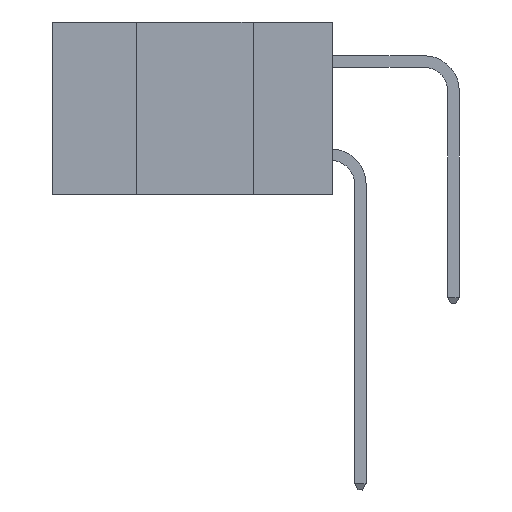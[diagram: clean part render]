
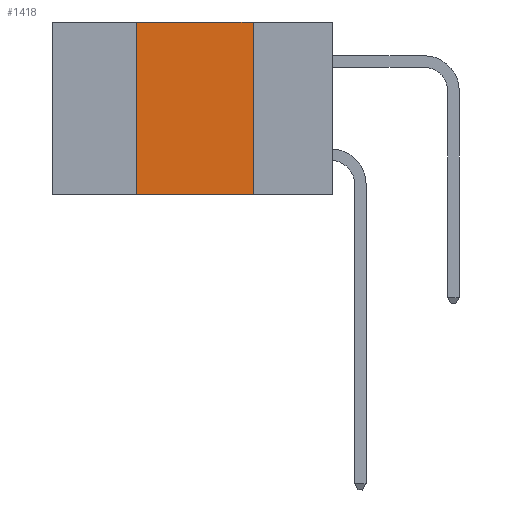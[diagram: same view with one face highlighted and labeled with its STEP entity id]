
A CAD part, left-side view. The second image highlights one B-rep face of the part: STEP entity #1418.
In plain terms, the highlighted planar face has unit normal (-1, 0, 0).
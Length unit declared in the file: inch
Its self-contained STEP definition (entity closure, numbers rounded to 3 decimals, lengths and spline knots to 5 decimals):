
#689 = ORIENTED_EDGE ( 'NONE', *, *, #16789, .F. ) ;
#822 = EDGE_CURVE ( 'NONE', #5186, #8439, #10412, .T. ) ;
#1418 = ADVANCED_FACE ( 'NONE', ( #10681 ), #15147, .F. ) ;
#1556 = ORIENTED_EDGE ( 'NONE', *, *, #2666, .T. ) ;
#1690 = DIRECTION ( 'NONE',  ( 1., 0., 0. ) ) ;
#2084 = LINE ( 'NONE', #8183, #17464 ) ;
#2623 = DIRECTION ( 'NONE',  ( 0., 0., -1. ) ) ;
#2666 = EDGE_CURVE ( 'NONE', #4254, #8439, #4034, .T. ) ;
#2769 = DIRECTION ( 'NONE',  ( 0., -1., 0. ) ) ;
#3243 = EDGE_LOOP ( 'NONE', ( #11813, #689, #13471, #1556 ) ) ;
#4034 = LINE ( 'NONE', #10139, #12313 ) ;
#4254 = VERTEX_POINT ( 'NONE', #14748 ) ;
#4379 = VECTOR ( 'NONE', #8027, 39.37008 ) ;
#4382 = VERTEX_POINT ( 'NONE', #11954 ) ;
#4491 = DIRECTION ( 'NONE',  ( 0., 0., -1. ) ) ;
#5186 = VERTEX_POINT ( 'NONE', #17676 ) ;
#7497 = AXIS2_PLACEMENT_3D ( 'NONE', #18267, #1690, #4491 ) ;
#8027 = DIRECTION ( 'NONE',  ( 0., 0., 1. ) ) ;
#8183 = CARTESIAN_POINT ( 'NONE',  ( 0., 0.6, 0. ) ) ;
#8439 = VERTEX_POINT ( 'NONE', #12436 ) ;
#10111 = CARTESIAN_POINT ( 'NONE',  ( 0., 0.17, -0.37 ) ) ;
#10139 = CARTESIAN_POINT ( 'NONE',  ( 0., 0.6, -0.37 ) ) ;
#10229 = EDGE_CURVE ( 'NONE', #4254, #4382, #13881, .T. ) ;
#10412 = LINE ( 'NONE', #10111, #13790 ) ;
#10681 = FACE_OUTER_BOUND ( 'NONE', #3243, .T. ) ;
#11813 = ORIENTED_EDGE ( 'NONE', *, *, #822, .F. ) ;
#11954 = CARTESIAN_POINT ( 'NONE',  ( 0., 0.42, 0. ) ) ;
#12313 = VECTOR ( 'NONE', #14716, 39.37008 ) ;
#12436 = CARTESIAN_POINT ( 'NONE',  ( 0., 0.17, -0.37 ) ) ;
#12508 = CARTESIAN_POINT ( 'NONE',  ( 0., 0.42, -0.37 ) ) ;
#13471 = ORIENTED_EDGE ( 'NONE', *, *, #10229, .F. ) ;
#13790 = VECTOR ( 'NONE', #2623, 39.37008 ) ;
#13881 = LINE ( 'NONE', #12508, #4379 ) ;
#14716 = DIRECTION ( 'NONE',  ( 0., -1., 0. ) ) ;
#14748 = CARTESIAN_POINT ( 'NONE',  ( 0., 0.42, -0.37 ) ) ;
#15147 = PLANE ( 'NONE',  #7497 ) ;
#16789 = EDGE_CURVE ( 'NONE', #4382, #5186, #2084, .T. ) ;
#17464 = VECTOR ( 'NONE', #2769, 39.37008 ) ;
#17676 = CARTESIAN_POINT ( 'NONE',  ( 0., 0.17, 0. ) ) ;
#18267 = CARTESIAN_POINT ( 'NONE',  ( 0., 0.6, 0. ) ) ;
